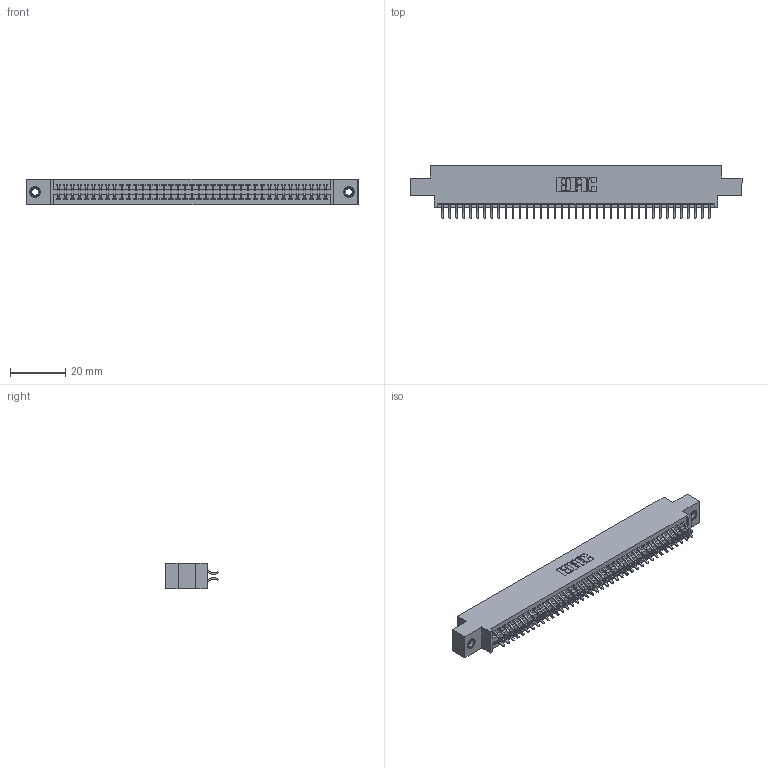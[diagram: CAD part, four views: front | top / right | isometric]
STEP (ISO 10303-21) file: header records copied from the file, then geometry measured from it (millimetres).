
FILE_DESCRIPTION (( 'STEP AP203' ), '1' );
FILE_NAME ('395-078-556-807.STEP', '2018-11-28T01:46:02', ( '' ), ( '' ), 'SwSTEP 2.0', 'SolidWorks 2016', '' );
FILE_SCHEMA (( 'CONFIG_CONTROL_DESIGN' ));
Length unit declared in the file: inch
Products named in the file (4): 345 Part_0.170 Offset - 0.156 Dia-TI; 345-292-001_556 Tail; 395-078-556-807; 345-250-001_345-250-005-103
Assembly tree (81 placements, depth 2):
  395-078-556-807
    345 Part_0.170 Offset - 0.156 Dia-TI
    345-292-001_556 Tail  x78
    345-250-001_345-250-005-103  x2
Bounding box: 120.27 x 19.24 x 9.4 mm (x, y, z)
Volume: 11525.2 mm3; surface area: 17081.2 mm2
Topology: 81 solids, 81 shells, 4558 faces, 13515 edges, 8898 vertices
Faces by surface type: plane 3002, cylinder 1540, cone 12, torus 4
Entity records: 32542 total; most frequent: CARTESIAN_POINT 5455, ORIENTED_EDGE 5370, DIRECTION 4827, EDGE_CURVE 2685, VECTOR 2369, LINE 2369, VERTEX_POINT 1784, AXIS2_PLACEMENT_3D 1229
